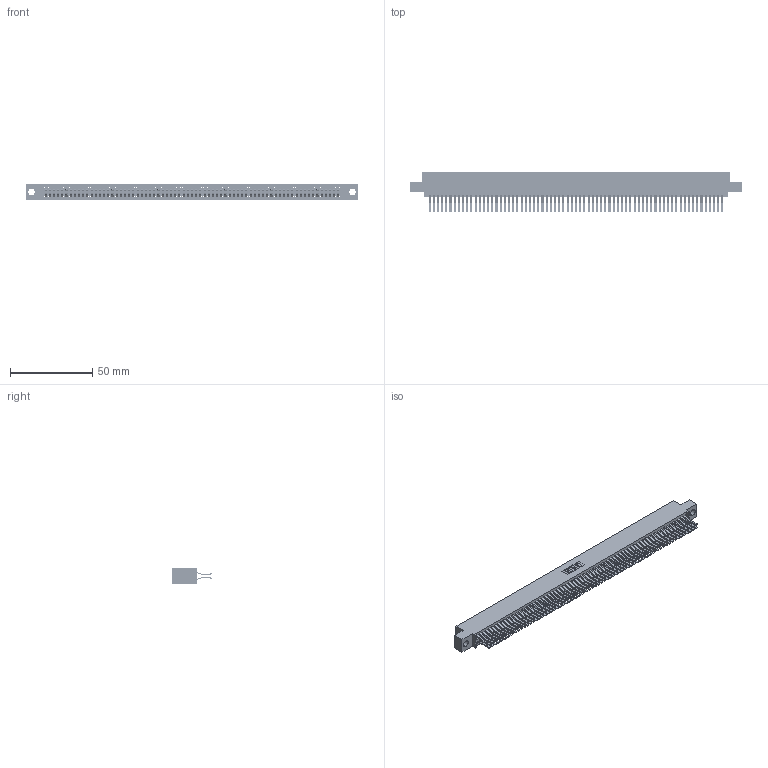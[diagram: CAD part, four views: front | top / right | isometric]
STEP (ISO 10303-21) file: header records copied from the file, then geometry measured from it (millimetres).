
FILE_DESCRIPTION (( 'STEP AP203' ), '1' );
FILE_NAME ('345-142-560-504.STEP', '2021-05-26T02:27:44', ( '' ), ( '' ), 'SwSTEP 2.0', 'SolidWorks 2020', '' );
FILE_SCHEMA (( 'CONFIG_CONTROL_DESIGN' ));
Length unit declared in the file: inch
Products named in the file (3): 345-292-001_560 Tail; 345-142-560-504; 345 Part_0.110 Offset - 0.156 Dia-TI
Assembly tree (143 placements, depth 2):
  345-142-560-504
    345 Part_0.110 Offset - 0.156 Dia-TI
    345-292-001_560 Tail  x142
Bounding box: 201.55 x 24.45 x 9.4 mm (x, y, z)
Volume: 20599.3 mm3; surface area: 33349.1 mm2
Topology: 143 solids, 143 shells, 7528 faces, 22399 edges, 14742 vertices
Faces by surface type: plane 4784, cylinder 2744
Entity records: 52443 total; most frequent: CARTESIAN_POINT 8770, ORIENTED_EDGE 8702, DIRECTION 7699, EDGE_CURVE 4351, VECTOR 3931, LINE 3931, VERTEX_POINT 2898, AXIS2_PLACEMENT_3D 1884
